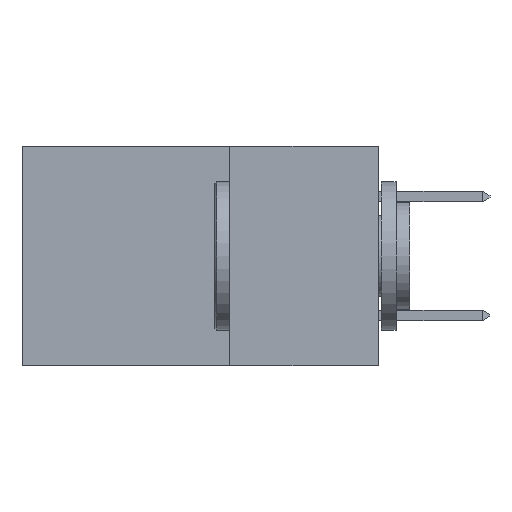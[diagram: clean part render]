
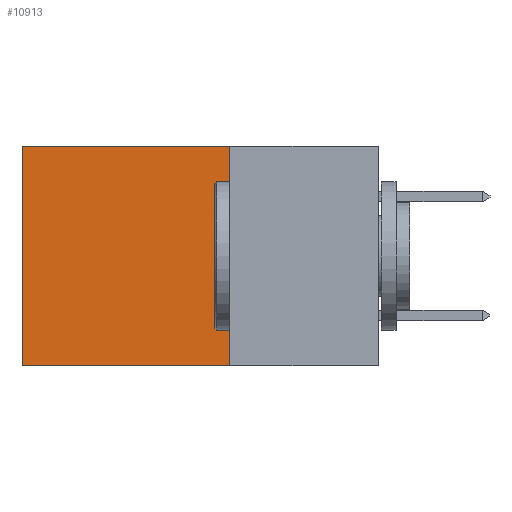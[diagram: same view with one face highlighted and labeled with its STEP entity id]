
A CAD part, left-side view. The second image highlights one B-rep face of the part: STEP entity #10913.
In plain terms, the highlighted planar face has unit normal (-1, 0, 0).
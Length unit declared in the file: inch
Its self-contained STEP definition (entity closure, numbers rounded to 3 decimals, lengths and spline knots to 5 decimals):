
#222 = VECTOR ( 'NONE', #10977, 39.37008 ) ;
#1510 = DIRECTION ( 'NONE',  ( 1., 0., 0. ) ) ;
#1536 = CARTESIAN_POINT ( 'NONE',  ( 0.298, 0.25, 0. ) ) ;
#1743 = DIRECTION ( 'NONE',  ( 0., 0., -1. ) ) ;
#1872 = EDGE_CURVE ( 'NONE', #6254, #8943, #3440, .T. ) ;
#2214 = LINE ( 'NONE', #14067, #11607 ) ;
#2233 = CARTESIAN_POINT ( 'NONE',  ( 0.298, 0.25, 0. ) ) ;
#3440 = LINE ( 'NONE', #6154, #222 ) ;
#4397 = EDGE_LOOP ( 'NONE', ( #12388, #6858, #14580, #7678 ) ) ;
#4940 = VECTOR ( 'NONE', #9580, 39.37008 ) ;
#5023 = CARTESIAN_POINT ( 'NONE',  ( 0.298, 0.25, -0.37 ) ) ;
#6154 = CARTESIAN_POINT ( 'NONE',  ( 0.298, 0.25, -0.37 ) ) ;
#6254 = VERTEX_POINT ( 'NONE', #5023 ) ;
#6379 = CARTESIAN_POINT ( 'NONE',  ( 0.298, 0.25, 0. ) ) ;
#6559 = VERTEX_POINT ( 'NONE', #6847 ) ;
#6847 = CARTESIAN_POINT ( 'NONE',  ( 0.298, 0.6, 0. ) ) ;
#6858 = ORIENTED_EDGE ( 'NONE', *, *, #1872, .F. ) ;
#7231 = AXIS2_PLACEMENT_3D ( 'NONE', #6379, #1510, #10078 ) ;
#7678 = ORIENTED_EDGE ( 'NONE', *, *, #11858, .T. ) ;
#7735 = EDGE_CURVE ( 'NONE', #8344, #6254, #2214, .T. ) ;
#8055 = VECTOR ( 'NONE', #12614, 39.37008 ) ;
#8344 = VERTEX_POINT ( 'NONE', #1536 ) ;
#8460 = LINE ( 'NONE', #11350, #8055 ) ;
#8856 = PLANE ( 'NONE',  #7231 ) ;
#8943 = VERTEX_POINT ( 'NONE', #12100 ) ;
#9580 = DIRECTION ( 'NONE',  ( 0., 1., 0. ) ) ;
#10078 = DIRECTION ( 'NONE',  ( 0., 0., -1. ) ) ;
#10913 = ADVANCED_FACE ( 'NONE', ( #13908 ), #8856, .F. ) ;
#10977 = DIRECTION ( 'NONE',  ( 0., 1., 0. ) ) ;
#11350 = CARTESIAN_POINT ( 'NONE',  ( 0.298, 0.6, 0. ) ) ;
#11489 = LINE ( 'NONE', #2233, #4940 ) ;
#11607 = VECTOR ( 'NONE', #1743, 39.37008 ) ;
#11858 = EDGE_CURVE ( 'NONE', #8344, #6559, #11489, .T. ) ;
#12100 = CARTESIAN_POINT ( 'NONE',  ( 0.298, 0.6, -0.37 ) ) ;
#12388 = ORIENTED_EDGE ( 'NONE', *, *, #13649, .T. ) ;
#12614 = DIRECTION ( 'NONE',  ( 0., 0., -1. ) ) ;
#13649 = EDGE_CURVE ( 'NONE', #6559, #8943, #8460, .T. ) ;
#13908 = FACE_OUTER_BOUND ( 'NONE', #4397, .T. ) ;
#14067 = CARTESIAN_POINT ( 'NONE',  ( 0.298, 0.25, 0. ) ) ;
#14580 = ORIENTED_EDGE ( 'NONE', *, *, #7735, .F. ) ;
